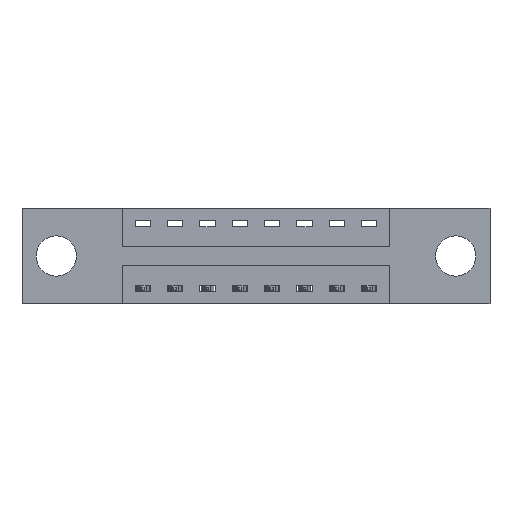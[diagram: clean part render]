
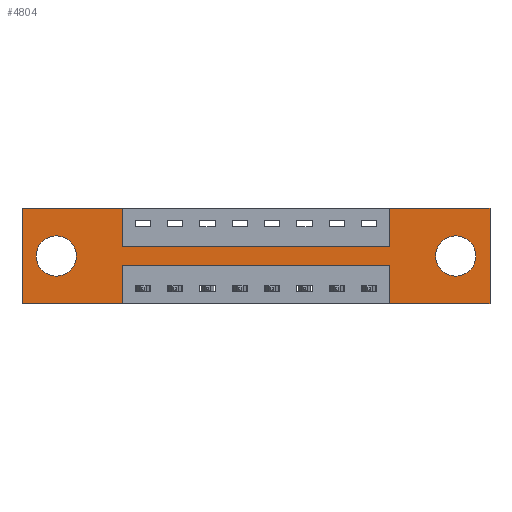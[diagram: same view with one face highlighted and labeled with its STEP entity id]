
A CAD part, front view. The second image highlights one B-rep face of the part: STEP entity #4804.
In plain terms, the highlighted planar face has unit normal (0, -1, 0).
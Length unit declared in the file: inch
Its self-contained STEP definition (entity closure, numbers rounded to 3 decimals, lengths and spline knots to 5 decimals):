
#248 = EDGE_CURVE ( 'NONE', #4442, #612, #8938, .T. ) ;
#348 = CARTESIAN_POINT ( 'NONE',  ( 0., 0., -0.37 ) ) ;
#460 = EDGE_CURVE ( 'NONE', #594, #1788, #6518, .T. ) ;
#503 = AXIS2_PLACEMENT_3D ( 'NONE', #7354, #3178, #8082 ) ;
#561 = ORIENTED_EDGE ( 'NONE', *, *, #248, .F. ) ;
#575 = ORIENTED_EDGE ( 'NONE', *, *, #8354, .F. ) ;
#594 = VERTEX_POINT ( 'NONE', #5976 ) ;
#612 = VERTEX_POINT ( 'NONE', #4418 ) ;
#822 = EDGE_CURVE ( 'NONE', #4231, #8771, #5633, .T. ) ;
#1183 = CARTESIAN_POINT ( 'NONE',  ( 1.6775, 0., -0.263 ) ) ;
#1256 = CARTESIAN_POINT ( 'NONE',  ( 0.3875, 0., -0.15 ) ) ;
#1320 = VECTOR ( 'NONE', #6345, 39.37008 ) ;
#1369 = EDGE_CURVE ( 'NONE', #3225, #7104, #2408, .T. ) ;
#1440 = CARTESIAN_POINT ( 'NONE',  ( 0.3875, 0., -0.15 ) ) ;
#1543 = EDGE_CURVE ( 'NONE', #1788, #594, #7956, .T. ) ;
#1546 = CARTESIAN_POINT ( 'NONE',  ( 1.4225, 0., -0.37 ) ) ;
#1788 = VERTEX_POINT ( 'NONE', #6173 ) ;
#1882 = EDGE_CURVE ( 'NONE', #6315, #3225, #7628, .T. ) ;
#1957 = ORIENTED_EDGE ( 'NONE', *, *, #4779, .F. ) ;
#1974 = EDGE_CURVE ( 'NONE', #2913, #4231, #8846, .T. ) ;
#1989 = DIRECTION ( 'NONE',  ( -1., 0., 0. ) ) ;
#2007 = VECTOR ( 'NONE', #6838, 39.37008 ) ;
#2020 = CARTESIAN_POINT ( 'NONE',  ( 0., 0., 0. ) ) ;
#2037 = LINE ( 'NONE', #2591, #5652 ) ;
#2321 = AXIS2_PLACEMENT_3D ( 'NONE', #7185, #2975, #7907 ) ;
#2329 = ORIENTED_EDGE ( 'NONE', *, *, #1882, .F. ) ;
#2408 = LINE ( 'NONE', #7754, #6228 ) ;
#2591 = CARTESIAN_POINT ( 'NONE',  ( 0.3875, 0., -0.37 ) ) ;
#2740 = DIRECTION ( 'NONE',  ( 0., 0., 1. ) ) ;
#2764 = CARTESIAN_POINT ( 'NONE',  ( 1.81, 0., 0. ) ) ;
#2859 = CARTESIAN_POINT ( 'NONE',  ( 0., 0., -0.37 ) ) ;
#2860 = LINE ( 'NONE', #6280, #6198 ) ;
#2875 = CARTESIAN_POINT ( 'NONE',  ( 1.81, 0., -0.37 ) ) ;
#2908 = EDGE_CURVE ( 'NONE', #9332, #5884, #4552, .T. ) ;
#2913 = VERTEX_POINT ( 'NONE', #1440 ) ;
#2949 = CARTESIAN_POINT ( 'NONE',  ( 1.4225, 0., 0. ) ) ;
#2975 = DIRECTION ( 'NONE',  ( 0., 1., 0. ) ) ;
#3055 = CARTESIAN_POINT ( 'NONE',  ( 1.6775, 0., -0.185 ) ) ;
#3178 = DIRECTION ( 'NONE',  ( 0., 1., 0. ) ) ;
#3183 = AXIS2_PLACEMENT_3D ( 'NONE', #4216, #4708, #4301 ) ;
#3213 = CARTESIAN_POINT ( 'NONE',  ( 1.4225, 0., -0.37 ) ) ;
#3225 = VERTEX_POINT ( 'NONE', #9578 ) ;
#3227 = VECTOR ( 'NONE', #6373, 39.37008 ) ;
#3234 = CARTESIAN_POINT ( 'NONE',  ( 1.4225, 0., 0. ) ) ;
#3272 = AXIS2_PLACEMENT_3D ( 'NONE', #348, #7751, #3558 ) ;
#3374 = LINE ( 'NONE', #2764, #1320 ) ;
#3419 = VERTEX_POINT ( 'NONE', #3701 ) ;
#3448 = ORIENTED_EDGE ( 'NONE', *, *, #8511, .F. ) ;
#3478 = DIRECTION ( 'NONE',  ( -1., 0., 0. ) ) ;
#3527 = FACE_BOUND ( 'NONE', #4091, .T. ) ;
#3558 = DIRECTION ( 'NONE',  ( 0., 0., -1. ) ) ;
#3647 = EDGE_CURVE ( 'NONE', #6784, #6315, #8367, .T. ) ;
#3684 = ORIENTED_EDGE ( 'NONE', *, *, #8052, .T. ) ;
#3701 = CARTESIAN_POINT ( 'NONE',  ( 1.81, 0., 0. ) ) ;
#3755 = LINE ( 'NONE', #5601, #7237 ) ;
#3784 = DIRECTION ( 'NONE',  ( 0., 0., -1. ) ) ;
#4081 = DIRECTION ( 'NONE',  ( 0., 0., -1. ) ) ;
#4091 = EDGE_LOOP ( 'NONE', ( #3684, #6139 ) ) ;
#4216 = CARTESIAN_POINT ( 'NONE',  ( 0.1325, 0., -0.185 ) ) ;
#4231 = VERTEX_POINT ( 'NONE', #6543 ) ;
#4301 = DIRECTION ( 'NONE',  ( 0., 0., 1. ) ) ;
#4306 = VECTOR ( 'NONE', #7836, 39.37008 ) ;
#4418 = CARTESIAN_POINT ( 'NONE',  ( 1.4225, 0., -0.22 ) ) ;
#4442 = VERTEX_POINT ( 'NONE', #3213 ) ;
#4552 = CIRCLE ( 'NONE', #2321, 0.078 ) ;
#4708 = DIRECTION ( 'NONE',  ( 0., 1., 0. ) ) ;
#4779 = EDGE_CURVE ( 'NONE', #8771, #3419, #7452, .T. ) ;
#4804 = ADVANCED_FACE ( 'NONE', ( #3527, #5629, #7016 ), #7032, .T. ) ;
#4915 = EDGE_CURVE ( 'NONE', #7104, #2913, #8014, .T. ) ;
#4916 = ORIENTED_EDGE ( 'NONE', *, *, #1974, .F. ) ;
#5208 = VECTOR ( 'NONE', #8958, 39.37008 ) ;
#5302 = CARTESIAN_POINT ( 'NONE',  ( 0., 0., -0.37 ) ) ;
#5305 = CARTESIAN_POINT ( 'NONE',  ( 1.6775, 0., -0.107 ) ) ;
#5340 = ORIENTED_EDGE ( 'NONE', *, *, #9292, .F. ) ;
#5601 = CARTESIAN_POINT ( 'NONE',  ( 0.3875, 0., -0.22 ) ) ;
#5629 = FACE_BOUND ( 'NONE', #6589, .T. ) ;
#5633 = LINE ( 'NONE', #3234, #2007 ) ;
#5652 = VECTOR ( 'NONE', #4081, 39.37008 ) ;
#5832 = ORIENTED_EDGE ( 'NONE', *, *, #1543, .T. ) ;
#5849 = ORIENTED_EDGE ( 'NONE', *, *, #7745, .F. ) ;
#5884 = VERTEX_POINT ( 'NONE', #5305 ) ;
#5976 = CARTESIAN_POINT ( 'NONE',  ( 0.1325, 0., -0.107 ) ) ;
#6126 = CARTESIAN_POINT ( 'NONE',  ( 0.3875, 0., -0.37 ) ) ;
#6139 = ORIENTED_EDGE ( 'NONE', *, *, #2908, .T. ) ;
#6173 = CARTESIAN_POINT ( 'NONE',  ( 0.1325, 0., -0.263 ) ) ;
#6198 = VECTOR ( 'NONE', #3478, 39.37008 ) ;
#6228 = VECTOR ( 'NONE', #6357, 39.37008 ) ;
#6276 = ORIENTED_EDGE ( 'NONE', *, *, #460, .T. ) ;
#6280 = CARTESIAN_POINT ( 'NONE',  ( 0., 0., -0.37 ) ) ;
#6301 = VECTOR ( 'NONE', #8069, 39.37008 ) ;
#6315 = VERTEX_POINT ( 'NONE', #2859 ) ;
#6325 = DIRECTION ( 'NONE',  ( 1., 0., 0. ) ) ;
#6345 = DIRECTION ( 'NONE',  ( 0., 0., -1. ) ) ;
#6357 = DIRECTION ( 'NONE',  ( 1., 0., 0. ) ) ;
#6373 = DIRECTION ( 'NONE',  ( 1., 0., 0. ) ) ;
#6410 = CARTESIAN_POINT ( 'NONE',  ( 0.3875, 0., 0. ) ) ;
#6518 = CIRCLE ( 'NONE', #3183, 0.078 ) ;
#6543 = CARTESIAN_POINT ( 'NONE',  ( 1.4225, 0., -0.15 ) ) ;
#6589 = EDGE_LOOP ( 'NONE', ( #6276, #5832 ) ) ;
#6768 = CIRCLE ( 'NONE', #7757, 0.078 ) ;
#6784 = VERTEX_POINT ( 'NONE', #6126 ) ;
#6828 = ORIENTED_EDGE ( 'NONE', *, *, #822, .F. ) ;
#6838 = DIRECTION ( 'NONE',  ( 0., 0., 1. ) ) ;
#6976 = EDGE_LOOP ( 'NONE', ( #575, #5340, #561, #3448, #5849, #1957, #6828, #4916, #8446, #9250, #2329, #7172 ) ) ;
#7016 = FACE_OUTER_BOUND ( 'NONE', #6976, .T. ) ;
#7032 = PLANE ( 'NONE',  #3272 ) ;
#7104 = VERTEX_POINT ( 'NONE', #6410 ) ;
#7122 = CARTESIAN_POINT ( 'NONE',  ( 0.3875, 0., 0. ) ) ;
#7172 = ORIENTED_EDGE ( 'NONE', *, *, #3647, .F. ) ;
#7185 = CARTESIAN_POINT ( 'NONE',  ( 1.6775, 0., -0.185 ) ) ;
#7237 = VECTOR ( 'NONE', #1989, 39.37008 ) ;
#7354 = CARTESIAN_POINT ( 'NONE',  ( 0.1325, 0., -0.185 ) ) ;
#7385 = VECTOR ( 'NONE', #2740, 39.37008 ) ;
#7452 = LINE ( 'NONE', #2020, #9133 ) ;
#7628 = LINE ( 'NONE', #7680, #7385 ) ;
#7680 = CARTESIAN_POINT ( 'NONE',  ( 0., 0., 0. ) ) ;
#7745 = EDGE_CURVE ( 'NONE', #3419, #9419, #3374, .T. ) ;
#7751 = DIRECTION ( 'NONE',  ( 0., -1., 0. ) ) ;
#7754 = CARTESIAN_POINT ( 'NONE',  ( 0., 0., 0. ) ) ;
#7757 = AXIS2_PLACEMENT_3D ( 'NONE', #3055, #7977, #3784 ) ;
#7836 = DIRECTION ( 'NONE',  ( 0., 0., -1. ) ) ;
#7907 = DIRECTION ( 'NONE',  ( 0., 0., -1. ) ) ;
#7956 = CIRCLE ( 'NONE', #503, 0.078 ) ;
#7977 = DIRECTION ( 'NONE',  ( 0., 1., 0. ) ) ;
#8014 = LINE ( 'NONE', #7122, #4306 ) ;
#8052 = EDGE_CURVE ( 'NONE', #5884, #9332, #6768, .T. ) ;
#8069 = DIRECTION ( 'NONE',  ( -1., 0., 0. ) ) ;
#8082 = DIRECTION ( 'NONE',  ( 0., 0., 1. ) ) ;
#8350 = CARTESIAN_POINT ( 'NONE',  ( 0.3875, 0., -0.22 ) ) ;
#8354 = EDGE_CURVE ( 'NONE', #8510, #6784, #2037, .T. ) ;
#8367 = LINE ( 'NONE', #5302, #6301 ) ;
#8446 = ORIENTED_EDGE ( 'NONE', *, *, #4915, .F. ) ;
#8510 = VERTEX_POINT ( 'NONE', #8350 ) ;
#8511 = EDGE_CURVE ( 'NONE', #9419, #4442, #2860, .T. ) ;
#8771 = VERTEX_POINT ( 'NONE', #2949 ) ;
#8846 = LINE ( 'NONE', #1256, #3227 ) ;
#8938 = LINE ( 'NONE', #1546, #5208 ) ;
#8958 = DIRECTION ( 'NONE',  ( 0., 0., 1. ) ) ;
#9133 = VECTOR ( 'NONE', #6325, 39.37008 ) ;
#9250 = ORIENTED_EDGE ( 'NONE', *, *, #1369, .F. ) ;
#9292 = EDGE_CURVE ( 'NONE', #612, #8510, #3755, .T. ) ;
#9332 = VERTEX_POINT ( 'NONE', #1183 ) ;
#9419 = VERTEX_POINT ( 'NONE', #2875 ) ;
#9578 = CARTESIAN_POINT ( 'NONE',  ( 0., 0., 0. ) ) ;
